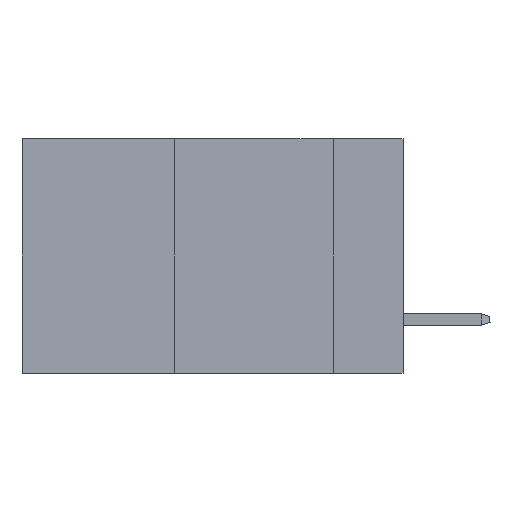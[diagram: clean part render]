
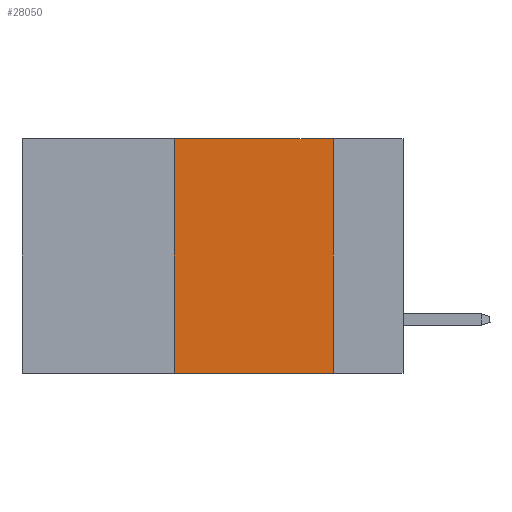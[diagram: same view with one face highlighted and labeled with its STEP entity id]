
A CAD part, left-side view. The second image highlights one B-rep face of the part: STEP entity #28050.
In plain terms, the highlighted planar face has unit normal (-1, 0, 0).
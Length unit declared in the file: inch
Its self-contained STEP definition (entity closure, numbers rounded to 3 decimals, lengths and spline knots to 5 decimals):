
#886 = CARTESIAN_POINT ( 'NONE',  ( 0., 0.11, -0.37 ) ) ;
#2316 = DIRECTION ( 'NONE',  ( 0., 0., 1. ) ) ;
#3070 = ORIENTED_EDGE ( 'NONE', *, *, #12258, .F. ) ;
#3450 = VERTEX_POINT ( 'NONE', #26807 ) ;
#4052 = EDGE_CURVE ( 'NONE', #3450, #19646, #31442, .T. ) ;
#5533 = CARTESIAN_POINT ( 'NONE',  ( 0., 0.6, 0. ) ) ;
#7282 = EDGE_CURVE ( 'NONE', #3450, #23417, #14212, .T. ) ;
#8599 = FACE_OUTER_BOUND ( 'NONE', #19438, .T. ) ;
#8802 = DIRECTION ( 'NONE',  ( 0., 0., -1. ) ) ;
#9177 = LINE ( 'NONE', #12046, #19620 ) ;
#9658 = EDGE_CURVE ( 'NONE', #23417, #13905, #9177, .T. ) ;
#10230 = LINE ( 'NONE', #35407, #14424 ) ;
#10921 = ORIENTED_EDGE ( 'NONE', *, *, #4052, .T. ) ;
#12046 = CARTESIAN_POINT ( 'NONE',  ( 0., 0.6, 0. ) ) ;
#12258 = EDGE_CURVE ( 'NONE', #13905, #19646, #10230, .T. ) ;
#12616 = CARTESIAN_POINT ( 'NONE',  ( 0., 0.6, -0.37 ) ) ;
#13680 = CARTESIAN_POINT ( 'NONE',  ( 0., 0.11, 0. ) ) ;
#13905 = VERTEX_POINT ( 'NONE', #13680 ) ;
#14212 = LINE ( 'NONE', #23836, #14232 ) ;
#14232 = VECTOR ( 'NONE', #2316, 39.37008 ) ;
#14424 = VECTOR ( 'NONE', #19666, 39.37008 ) ;
#19438 = EDGE_LOOP ( 'NONE', ( #3070, #27737, #23191, #10921 ) ) ;
#19620 = VECTOR ( 'NONE', #24553, 39.37008 ) ;
#19646 = VERTEX_POINT ( 'NONE', #886 ) ;
#19666 = DIRECTION ( 'NONE',  ( 0., 0., -1. ) ) ;
#19980 = CARTESIAN_POINT ( 'NONE',  ( 0., 0.36, 0. ) ) ;
#21123 = PLANE ( 'NONE',  #35082 ) ;
#21259 = VECTOR ( 'NONE', #37583, 39.37008 ) ;
#23191 = ORIENTED_EDGE ( 'NONE', *, *, #7282, .F. ) ;
#23417 = VERTEX_POINT ( 'NONE', #19980 ) ;
#23836 = CARTESIAN_POINT ( 'NONE',  ( 0., 0.36, 0. ) ) ;
#24553 = DIRECTION ( 'NONE',  ( 0., -1., 0. ) ) ;
#26807 = CARTESIAN_POINT ( 'NONE',  ( 0., 0.36, -0.37 ) ) ;
#27737 = ORIENTED_EDGE ( 'NONE', *, *, #9658, .F. ) ;
#28050 = ADVANCED_FACE ( 'NONE', ( #8599 ), #21123, .F. ) ;
#31332 = DIRECTION ( 'NONE',  ( 1., 0., 0. ) ) ;
#31442 = LINE ( 'NONE', #12616, #21259 ) ;
#35082 = AXIS2_PLACEMENT_3D ( 'NONE', #5533, #31332, #8802 ) ;
#35407 = CARTESIAN_POINT ( 'NONE',  ( 0., 0.11, 0. ) ) ;
#37583 = DIRECTION ( 'NONE',  ( 0., -1., 0. ) ) ;
